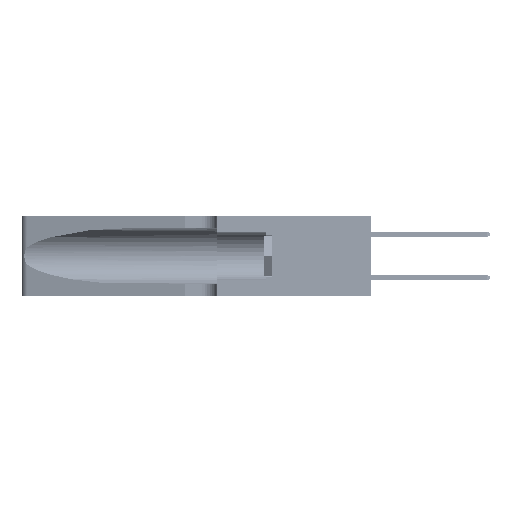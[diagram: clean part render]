
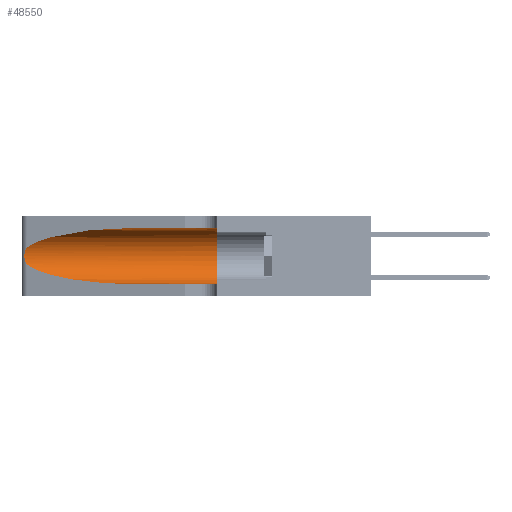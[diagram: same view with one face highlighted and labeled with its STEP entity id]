
A CAD part, left-side view. The second image highlights one B-rep face of the part: STEP entity #48550.
In plain terms, the highlighted cylindrical face has radius 3.308 mm (diameter 6.617 mm), a partial arc.
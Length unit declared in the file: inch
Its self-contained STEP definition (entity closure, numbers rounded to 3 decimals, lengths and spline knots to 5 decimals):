
#418 = EDGE_CURVE ( 'NONE', #29408, #26545, #15406, .T. ) ;
#694 = CARTESIAN_POINT ( 'NONE',  ( 0.25555, 1.22994, 0.2215 ) ) ;
#1702 = EDGE_CURVE ( 'NONE', #20704, #19990, #20071, .T. ) ;
#1881 = CARTESIAN_POINT ( 'NONE',  ( 0.25487, 1.22718, 0.14631 ) ) ;
#3054 = CARTESIAN_POINT ( 'NONE',  ( 0.25487, 1.22718, 0.14631 ) ) ;
#4041 = CARTESIAN_POINT ( 'NONE',  ( 0.1305, 1.61858, 0.185 ) ) ;
#4284 = CARTESIAN_POINT ( 'NONE',  ( 0.26017, 1.23833, 0.17102 ) ) ;
#6653 = CARTESIAN_POINT ( 'NONE',  ( 0.1305, 0.72297, 0.31525 ) ) ;
#7031 = CYLINDRICAL_SURFACE ( 'NONE', #16881, 0.13025 ) ;
#7224 = ORIENTED_EDGE ( 'NONE', *, *, #39533, .F. ) ;
#8248 = CARTESIAN_POINT ( 'NONE',  ( 0.26075, 1.23896, 0.178 ) ) ;
#11447 = CARTESIAN_POINT ( 'NONE',  ( 0.1305, 0.35, 0.185 ) ) ;
#12706 = AXIS2_PLACEMENT_3D ( 'NONE', #11447, #30290, #18974 ) ;
#13886 = DIRECTION ( 'NONE',  ( 0., -1., 0. ) ) ;
#15023 = VERTEX_POINT ( 'NONE', #38158 ) ;
#15152 = ORIENTED_EDGE ( 'NONE', *, *, #1702, .F. ) ;
#15164 = EDGE_CURVE ( 'NONE', #20704, #29408, #21398, .T. ) ;
#15406 = B_SPLINE_CURVE_WITH_KNOTS ( 'NONE', 3,
 ( #40300, #694, #44110, #20559, #23962, #47723, #27736, #8248, #4284, #31720, #43777, #35665, #20053, #35828 ),
 .UNSPECIFIED., .F., .F.,
 ( 4, 2, 2, 2, 2, 2, 4 ),
 ( 0., 0.00027, 0.00053, 0.00107, 0.0016, 0.00187, 0.00214 ),
 .UNSPECIFIED. ) ;
#16448 = LINE ( 'NONE', #43915, #26864 ) ;
#16881 = AXIS2_PLACEMENT_3D ( 'NONE', #4041, #19627, #36291 ) ;
#17435 = FACE_OUTER_BOUND ( 'NONE', #20509, .T. ) ;
#18482 = CARTESIAN_POINT ( 'NONE',  ( 0.1305, 0.72297, 0.05475 ) ) ;
#18974 = DIRECTION ( 'NONE',  ( 0., 0., 1. ) ) ;
#19627 = DIRECTION ( 'NONE',  ( 0., -1., 0. ) ) ;
#19990 = VERTEX_POINT ( 'NONE', #34140 ) ;
#20053 = CARTESIAN_POINT ( 'NONE',  ( 0.25555, 1.22993, 0.14849 ) ) ;
#20071 = LINE ( 'NONE', #37376, #50209 ) ;
#20509 = EDGE_LOOP ( 'NONE', ( #21109, #45455, #38372, #30765, #7224, #15152 ) ) ;
#20559 = CARTESIAN_POINT ( 'NONE',  ( 0.25787, 1.23484, 0.2124 ) ) ;
#20704 = VERTEX_POINT ( 'NONE', #6653 ) ;
#21109 = ORIENTED_EDGE ( 'NONE', *, *, #15164, .T. ) ;
#21398 =( BOUNDED_CURVE ( )  B_SPLINE_CURVE ( 3, ( #30139, #29640, #25506, #45313 ),
 .UNSPECIFIED., .F., .T. ) 
 B_SPLINE_CURVE_WITH_KNOTS ( ( 4, 4 ),
 ( 1.5708, 2.84003 ),
 .UNSPECIFIED. ) 
 CURVE ( )  GEOMETRIC_REPRESENTATION_ITEM ( )  RATIONAL_B_SPLINE_CURVE ( ( 1., 0.87, 0.87, 1. ) ) 
 REPRESENTATION_ITEM ( '' )  );
#23962 = CARTESIAN_POINT ( 'NONE',  ( 0.25854, 1.2359, 0.20912 ) ) ;
#25506 = CARTESIAN_POINT ( 'NONE',  ( 0.2373, 1.15595, 0.28018 ) ) ;
#26545 = VERTEX_POINT ( 'NONE', #1881 ) ;
#26673 = EDGE_CURVE ( 'NONE', #26545, #31765, #36820, .T. ) ;
#26864 = VECTOR ( 'NONE', #33037, 39.37008 ) ;
#27736 = CARTESIAN_POINT ( 'NONE',  ( 0.26075, 1.23896, 0.19203 ) ) ;
#28030 = EDGE_CURVE ( 'NONE', #31765, #15023, #16448, .T. ) ;
#29408 = VERTEX_POINT ( 'NONE', #45330 ) ;
#29640 = CARTESIAN_POINT ( 'NONE',  ( 0.18966, 0.96281, 0.31525 ) ) ;
#30139 = CARTESIAN_POINT ( 'NONE',  ( 0.1305, 0.72297, 0.31525 ) ) ;
#30290 = DIRECTION ( 'NONE',  ( 0., 1., 0. ) ) ;
#30765 = ORIENTED_EDGE ( 'NONE', *, *, #28030, .T. ) ;
#31720 = CARTESIAN_POINT ( 'NONE',  ( 0.25856, 1.23593, 0.16098 ) ) ;
#31765 = VERTEX_POINT ( 'NONE', #35777 ) ;
#32956 = CIRCLE ( 'NONE', #12706, 0.13025 ) ;
#33037 = DIRECTION ( 'NONE',  ( 0., -1., 0. ) ) ;
#34140 = CARTESIAN_POINT ( 'NONE',  ( 0.1305, 0.35, 0.31525 ) ) ;
#35665 = CARTESIAN_POINT ( 'NONE',  ( 0.25639, 1.23186, 0.15144 ) ) ;
#35777 = CARTESIAN_POINT ( 'NONE',  ( 0.1305, 0.72297, 0.05475 ) ) ;
#35828 = CARTESIAN_POINT ( 'NONE',  ( 0.25487, 1.22718, 0.14631 ) ) ;
#36291 = DIRECTION ( 'NONE',  ( 0., 0., -1. ) ) ;
#36820 =( BOUNDED_CURVE ( )  B_SPLINE_CURVE ( 3, ( #3054, #42011, #37691, #18482 ),
 .UNSPECIFIED., .F., .F. ) 
 B_SPLINE_CURVE_WITH_KNOTS ( ( 4, 4 ),
 ( 3.44316, 4.71239 ),
 .UNSPECIFIED. ) 
 CURVE ( )  GEOMETRIC_REPRESENTATION_ITEM ( )  RATIONAL_B_SPLINE_CURVE ( ( 1., 0.87, 0.87, 1. ) ) 
 REPRESENTATION_ITEM ( '' )  );
#37376 = CARTESIAN_POINT ( 'NONE',  ( 0.1305, 1.61858, 0.31525 ) ) ;
#37691 = CARTESIAN_POINT ( 'NONE',  ( 0.18966, 0.96281, 0.05475 ) ) ;
#38158 = CARTESIAN_POINT ( 'NONE',  ( 0.1305, 0.35, 0.05475 ) ) ;
#38372 = ORIENTED_EDGE ( 'NONE', *, *, #26673, .T. ) ;
#39533 = EDGE_CURVE ( 'NONE', #19990, #15023, #32956, .T. ) ;
#40300 = CARTESIAN_POINT ( 'NONE',  ( 0.25487, 1.22718, 0.22369 ) ) ;
#42011 = CARTESIAN_POINT ( 'NONE',  ( 0.2373, 1.15595, 0.08982 ) ) ;
#43777 = CARTESIAN_POINT ( 'NONE',  ( 0.25789, 1.23486, 0.15765 ) ) ;
#43915 = CARTESIAN_POINT ( 'NONE',  ( 0.1305, 1.61858, 0.05475 ) ) ;
#44110 = CARTESIAN_POINT ( 'NONE',  ( 0.25639, 1.23184, 0.21858 ) ) ;
#45313 = CARTESIAN_POINT ( 'NONE',  ( 0.25487, 1.22718, 0.22369 ) ) ;
#45330 = CARTESIAN_POINT ( 'NONE',  ( 0.25487, 1.22718, 0.22369 ) ) ;
#45455 = ORIENTED_EDGE ( 'NONE', *, *, #418, .T. ) ;
#47723 = CARTESIAN_POINT ( 'NONE',  ( 0.26018, 1.23835, 0.19895 ) ) ;
#48550 = ADVANCED_FACE ( 'NONE', ( #17435 ), #7031, .F. ) ;
#50209 = VECTOR ( 'NONE', #13886, 39.37008 ) ;
